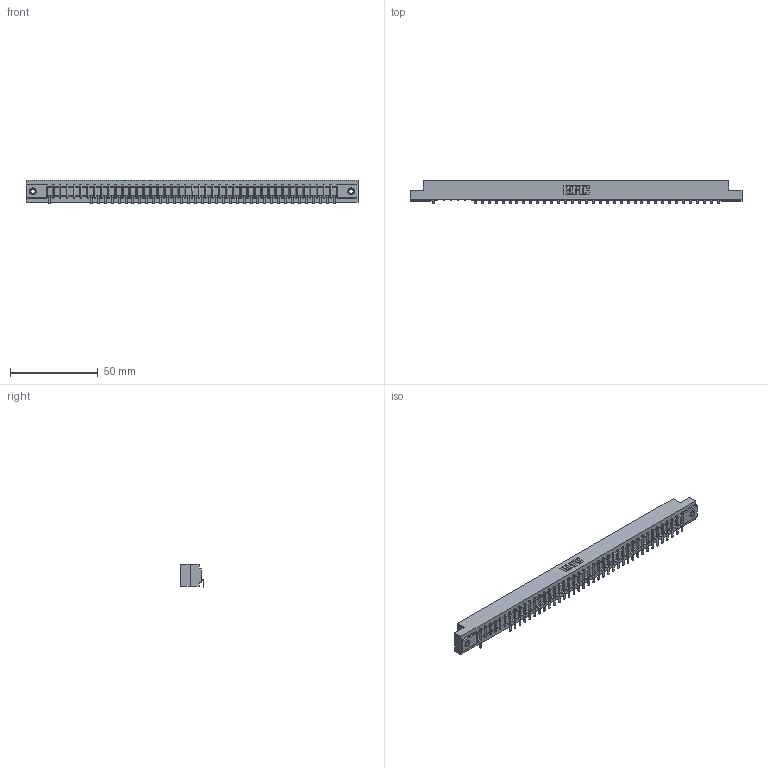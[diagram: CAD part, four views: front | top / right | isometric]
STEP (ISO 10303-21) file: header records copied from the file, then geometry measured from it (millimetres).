
FILE_DESCRIPTION (( 'STEP AP203' ), '1' );
FILE_NAME ('357-042-553-107.STEP', '2018-08-11T08:25:48', ( '' ), ( '' ), 'SwSTEP 2.0', 'SolidWorks 2016', '' );
FILE_SCHEMA (( 'CONFIG_CONTROL_DESIGN' ));
Length unit declared in the file: inch
Products named in the file (4): 307 Part_.156 Dia Mounting Holes; 307-290-002_553; 345-250-001_345-250-005-103; 357-042-553-107
Assembly tree (40 placements, depth 2):
  357-042-553-107
    307 Part_.156 Dia Mounting Holes
    307-290-002_553  x37
    345-250-001_345-250-005-103  x2
Bounding box: 189.43 x 13.32 x 13.5 mm (x, y, z)
Volume: 20113.4 mm3; surface area: 24389.3 mm2
Topology: 40 solids, 40 shells, 3207 faces, 9807 edges, 6414 vertices
Faces by surface type: plane 1901, cylinder 1204, sphere 86, cone 12, torus 4
Entity records: 37885 total; most frequent: CARTESIAN_POINT 6394, ORIENTED_EDGE 6382, DIRECTION 6217, EDGE_CURVE 3191, VECTOR 2443, LINE 2443, VERTEX_POINT 2064, AXIS2_PLACEMENT_3D 1887
